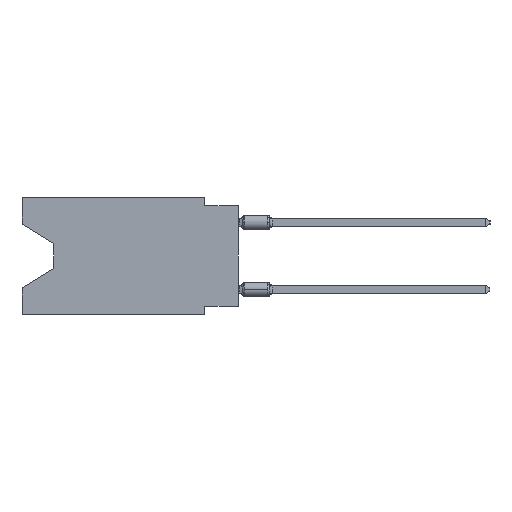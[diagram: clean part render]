
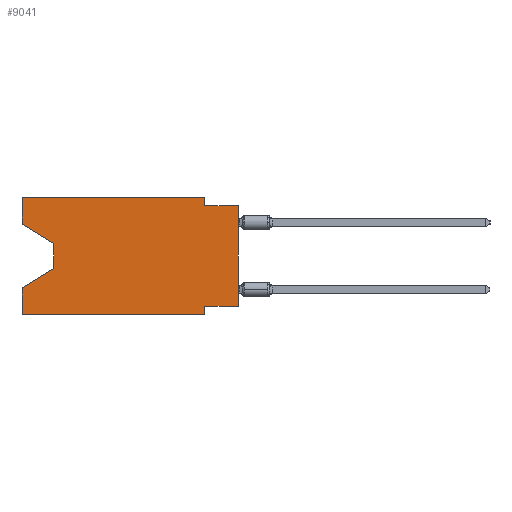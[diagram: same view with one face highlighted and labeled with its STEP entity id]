
A CAD part, left-side view. The second image highlights one B-rep face of the part: STEP entity #9041.
In plain terms, the highlighted planar face has unit normal (-1, 0, 0).
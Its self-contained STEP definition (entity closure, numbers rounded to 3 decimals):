
#331 = CARTESIAN_POINT ( 'NONE',  ( 0., 0., -0.635 ) ) ;
#781 = VECTOR ( 'NONE', #34287, 1000. ) ;
#849 = CARTESIAN_POINT ( 'NONE',  ( 0., 16.383, 0. ) ) ;
#1027 = CARTESIAN_POINT ( 'NONE',  ( 0., 16.383, 0. ) ) ;
#2358 = ORIENTED_EDGE ( 'NONE', *, *, #47676, .F. ) ;
#2580 = LINE ( 'NONE', #34316, #25694 ) ;
#2682 = VECTOR ( 'NONE', #33726, 1000. ) ;
#3059 = ORIENTED_EDGE ( 'NONE', *, *, #29465, .T. ) ;
#3671 = CARTESIAN_POINT ( 'NONE',  ( 0., 16.383, -8.89 ) ) ;
#3685 = EDGE_CURVE ( 'NONE', #44809, #13958, #41189, .T. ) ;
#3731 = DIRECTION ( 'NONE',  ( 0., 0., 1. ) ) ;
#4927 = ORIENTED_EDGE ( 'NONE', *, *, #28189, .F. ) ;
#5192 = VERTEX_POINT ( 'NONE', #32776 ) ;
#5417 = CARTESIAN_POINT ( 'NONE',  ( 0., 2.54, 0. ) ) ;
#6479 = EDGE_CURVE ( 'NONE', #42068, #36001, #35922, .T. ) ;
#6795 = CARTESIAN_POINT ( 'NONE',  ( 0., 16.383, 0. ) ) ;
#7584 = CARTESIAN_POINT ( 'NONE',  ( 0., 2.54, -8.89 ) ) ;
#8108 = DIRECTION ( 'NONE',  ( 0., 0., -1. ) ) ;
#8554 = VECTOR ( 'NONE', #27774, 1000. ) ;
#8872 = VECTOR ( 'NONE', #12790, 1000. ) ;
#8963 = CARTESIAN_POINT ( 'NONE',  ( 0., 0., -0.635 ) ) ;
#9041 = ADVANCED_FACE ( 'NONE', ( #30596 ), #26029, .F. ) ;
#9570 = EDGE_CURVE ( 'NONE', #38512, #26878, #39664, .T. ) ;
#9919 = CARTESIAN_POINT ( 'NONE',  ( 0., 16.383, -8.89 ) ) ;
#11479 = EDGE_CURVE ( 'NONE', #41083, #46398, #42886, .T. ) ;
#12534 = VECTOR ( 'NONE', #20552, 1000. ) ;
#12790 = DIRECTION ( 'NONE',  ( 0., -0.855, -0.519 ) ) ;
#13409 = DIRECTION ( 'NONE',  ( 0., -1., 0. ) ) ;
#13632 = VERTEX_POINT ( 'NONE', #34070 ) ;
#13958 = VERTEX_POINT ( 'NONE', #22236 ) ;
#15653 = VERTEX_POINT ( 'NONE', #50336 ) ;
#15836 = ORIENTED_EDGE ( 'NONE', *, *, #21404, .F. ) ;
#16452 = CARTESIAN_POINT ( 'NONE',  ( 0., 2.54, -8.255 ) ) ;
#16477 = CARTESIAN_POINT ( 'NONE',  ( 0., 13.97, -3.505 ) ) ;
#16804 = ORIENTED_EDGE ( 'NONE', *, *, #3685, .F. ) ;
#16898 = DIRECTION ( 'NONE',  ( 0., 0., 1. ) ) ;
#16999 = CARTESIAN_POINT ( 'NONE',  ( 0., 16.383, 0. ) ) ;
#18407 = CARTESIAN_POINT ( 'NONE',  ( 0., 2.54, 0. ) ) ;
#19089 = CARTESIAN_POINT ( 'NONE',  ( 0., 0., 0. ) ) ;
#20322 = EDGE_CURVE ( 'NONE', #21355, #15653, #50357, .T. ) ;
#20552 = DIRECTION ( 'NONE',  ( 0., 0., 1. ) ) ;
#20582 = LINE ( 'NONE', #16999, #38739 ) ;
#21355 = VERTEX_POINT ( 'NONE', #16452 ) ;
#21404 = EDGE_CURVE ( 'NONE', #13958, #46398, #35405, .T. ) ;
#21740 = CARTESIAN_POINT ( 'NONE',  ( 0., 0., -8.255 ) ) ;
#21903 = VECTOR ( 'NONE', #47415, 1000. ) ;
#21922 = AXIS2_PLACEMENT_3D ( 'NONE', #6795, #41623, #23173 ) ;
#22236 = CARTESIAN_POINT ( 'NONE',  ( 0., 2.54, -0.635 ) ) ;
#22615 = VECTOR ( 'NONE', #8108, 1000. ) ;
#23173 = DIRECTION ( 'NONE',  ( 0., 0., -1. ) ) ;
#25694 = VECTOR ( 'NONE', #45332, 1000. ) ;
#26029 = PLANE ( 'NONE',  #21922 ) ;
#26878 = VERTEX_POINT ( 'NONE', #48100 ) ;
#27774 = DIRECTION ( 'NONE',  ( 0., 0., -1. ) ) ;
#28133 = ORIENTED_EDGE ( 'NONE', *, *, #11479, .T. ) ;
#28189 = EDGE_CURVE ( 'NONE', #41083, #21355, #47649, .T. ) ;
#28735 = ORIENTED_EDGE ( 'NONE', *, *, #20322, .F. ) ;
#29465 = EDGE_CURVE ( 'NONE', #5192, #36001, #2580, .T. ) ;
#30596 = FACE_OUTER_BOUND ( 'NONE', #40266, .T. ) ;
#30878 = EDGE_CURVE ( 'NONE', #42068, #15653, #33221, .T. ) ;
#31795 = CARTESIAN_POINT ( 'NONE',  ( 0., 0., -8.255 ) ) ;
#32008 = ORIENTED_EDGE ( 'NONE', *, *, #9570, .T. ) ;
#32259 = LINE ( 'NONE', #1027, #42689 ) ;
#32353 = LINE ( 'NONE', #16477, #8554 ) ;
#32774 = EDGE_CURVE ( 'NONE', #26878, #5192, #32353, .T. ) ;
#32776 = CARTESIAN_POINT ( 'NONE',  ( 0., 13.97, -5.385 ) ) ;
#33221 = LINE ( 'NONE', #9919, #2682 ) ;
#33726 = DIRECTION ( 'NONE',  ( 0., -1., 0. ) ) ;
#34070 = CARTESIAN_POINT ( 'NONE',  ( 0., 16.383, 0. ) ) ;
#34121 = VECTOR ( 'NONE', #3731, 1000. ) ;
#34143 = EDGE_CURVE ( 'NONE', #13632, #44809, #20582, .T. ) ;
#34287 = DIRECTION ( 'NONE',  ( 0., 0., -1. ) ) ;
#34316 = CARTESIAN_POINT ( 'NONE',  ( 0., 13.97, -5.385 ) ) ;
#35405 = LINE ( 'NONE', #331, #37410 ) ;
#35922 = LINE ( 'NONE', #849, #12534 ) ;
#36001 = VERTEX_POINT ( 'NONE', #42998 ) ;
#37410 = VECTOR ( 'NONE', #47202, 1000. ) ;
#38512 = VERTEX_POINT ( 'NONE', #47612 ) ;
#38739 = VECTOR ( 'NONE', #13409, 1000. ) ;
#39664 = LINE ( 'NONE', #40679, #8872 ) ;
#40266 = EDGE_LOOP ( 'NONE', ( #32008, #44849, #3059, #41723, #50060, #28735, #4927, #28133, #15836, #16804, #40793, #2358 ) ) ;
#40679 = CARTESIAN_POINT ( 'NONE',  ( 0., 16.383, -2.038 ) ) ;
#40793 = ORIENTED_EDGE ( 'NONE', *, *, #34143, .F. ) ;
#41083 = VERTEX_POINT ( 'NONE', #21740 ) ;
#41189 = LINE ( 'NONE', #18407, #781 ) ;
#41623 = DIRECTION ( 'NONE',  ( 1., 0., 0. ) ) ;
#41723 = ORIENTED_EDGE ( 'NONE', *, *, #6479, .F. ) ;
#42068 = VERTEX_POINT ( 'NONE', #3671 ) ;
#42689 = VECTOR ( 'NONE', #16898, 1000. ) ;
#42886 = LINE ( 'NONE', #19089, #34121 ) ;
#42998 = CARTESIAN_POINT ( 'NONE',  ( 0., 16.383, -6.852 ) ) ;
#44809 = VERTEX_POINT ( 'NONE', #5417 ) ;
#44849 = ORIENTED_EDGE ( 'NONE', *, *, #32774, .T. ) ;
#45332 = DIRECTION ( 'NONE',  ( 0., 0.855, -0.519 ) ) ;
#46398 = VERTEX_POINT ( 'NONE', #8963 ) ;
#47202 = DIRECTION ( 'NONE',  ( 0., -1., 0. ) ) ;
#47415 = DIRECTION ( 'NONE',  ( 0., 1., 0. ) ) ;
#47612 = CARTESIAN_POINT ( 'NONE',  ( 0., 16.383, -2.038 ) ) ;
#47649 = LINE ( 'NONE', #31795, #21903 ) ;
#47676 = EDGE_CURVE ( 'NONE', #38512, #13632, #32259, .T. ) ;
#48100 = CARTESIAN_POINT ( 'NONE',  ( 0., 13.97, -3.505 ) ) ;
#50060 = ORIENTED_EDGE ( 'NONE', *, *, #30878, .T. ) ;
#50336 = CARTESIAN_POINT ( 'NONE',  ( 0., 2.54, -8.89 ) ) ;
#50357 = LINE ( 'NONE', #7584, #22615 ) ;
